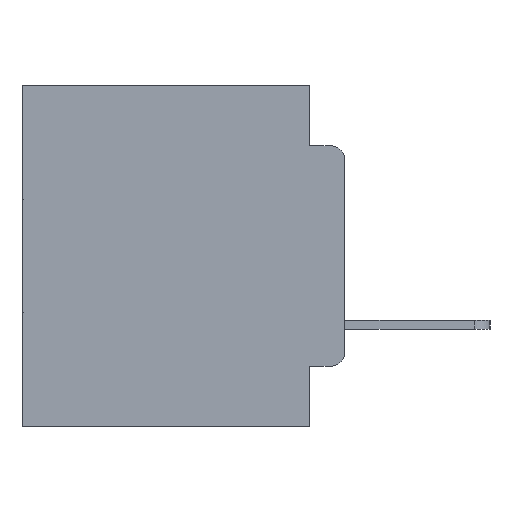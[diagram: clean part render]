
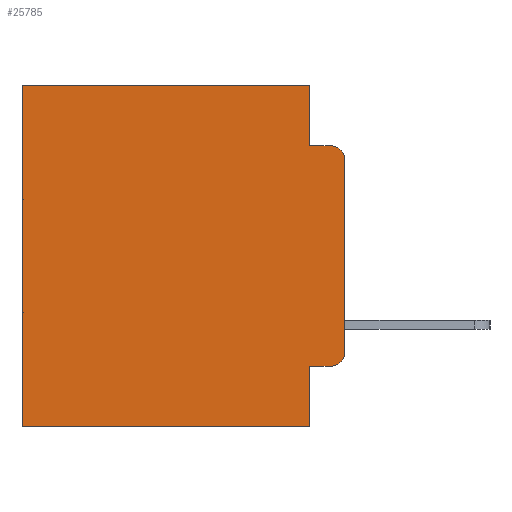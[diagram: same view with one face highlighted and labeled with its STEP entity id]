
A CAD part, left-side view. The second image highlights one B-rep face of the part: STEP entity #25785.
In plain terms, the highlighted planar face has unit normal (-1, 0, 0).
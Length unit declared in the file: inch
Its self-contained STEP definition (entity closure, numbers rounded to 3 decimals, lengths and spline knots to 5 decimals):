
#157 = CARTESIAN_POINT ( 'NONE',  ( 0.298, 0., -0.3915 ) ) ;
#296 = AXIS2_PLACEMENT_3D ( 'NONE', #23354, #9977, #25510 ) ;
#390 = DIRECTION ( 'NONE',  ( 1., 0., 0. ) ) ;
#1277 = LINE ( 'NONE', #17459, #25351 ) ;
#1589 = DIRECTION ( 'NONE',  ( 0., -1., 0. ) ) ;
#1739 = LINE ( 'NONE', #18466, #7042 ) ;
#2815 = ORIENTED_EDGE ( 'NONE', *, *, #13918, .F. ) ;
#3481 = FACE_OUTER_BOUND ( 'NONE', #18692, .T. ) ;
#3540 = CARTESIAN_POINT ( 'NONE',  ( 0.298, 0.051, 0. ) ) ;
#3542 = EDGE_CURVE ( 'NONE', #17541, #8815, #22103, .T. ) ;
#3985 = ORIENTED_EDGE ( 'NONE', *, *, #18609, .T. ) ;
#4262 = ORIENTED_EDGE ( 'NONE', *, *, #20008, .F. ) ;
#4899 = ORIENTED_EDGE ( 'NONE', *, *, #21654, .F. ) ;
#5391 = CARTESIAN_POINT ( 'NONE',  ( 0.298, 0.02, -0.1085 ) ) ;
#5710 = ORIENTED_EDGE ( 'NONE', *, *, #10052, .T. ) ;
#6022 = LINE ( 'NONE', #25592, #12409 ) ;
#6202 = ORIENTED_EDGE ( 'NONE', *, *, #3542, .T. ) ;
#6650 = ORIENTED_EDGE ( 'NONE', *, *, #12881, .F. ) ;
#7029 = ORIENTED_EDGE ( 'NONE', *, *, #26324, .F. ) ;
#7042 = VECTOR ( 'NONE', #18252, 39.37008 ) ;
#7412 = ORIENTED_EDGE ( 'NONE', *, *, #27875, .T. ) ;
#7797 = ORIENTED_EDGE ( 'NONE', *, *, #28250, .T. ) ;
#7899 = DIRECTION ( 'NONE',  ( 0., 0., -1. ) ) ;
#8348 = CARTESIAN_POINT ( 'NONE',  ( 0.298, 0., -0.5 ) ) ;
#8815 = VERTEX_POINT ( 'NONE', #25497 ) ;
#8948 = VERTEX_POINT ( 'NONE', #21091 ) ;
#9608 = AXIS2_PLACEMENT_3D ( 'NONE', #5391, #21474, #7899 ) ;
#9977 = DIRECTION ( 'NONE',  ( -1., 0., 0. ) ) ;
#10052 = EDGE_CURVE ( 'NONE', #25982, #17541, #1739, .T. ) ;
#10218 = VECTOR ( 'NONE', #15419, 39.37008 ) ;
#10596 = CARTESIAN_POINT ( 'NONE',  ( 0.298, 0., 0. ) ) ;
#10712 = CARTESIAN_POINT ( 'NONE',  ( 0.298, 0.02, -0.4115 ) ) ;
#10760 = DIRECTION ( 'NONE',  ( 0., 1., 0. ) ) ;
#11205 = VECTOR ( 'NONE', #17823, 39.37008 ) ;
#11633 = CARTESIAN_POINT ( 'NONE',  ( 0.298, 0.02, -0.0885 ) ) ;
#11638 = VERTEX_POINT ( 'NONE', #27804 ) ;
#12241 = CARTESIAN_POINT ( 'NONE',  ( 0.298, 0.051, -0.5 ) ) ;
#12368 = VERTEX_POINT ( 'NONE', #157 ) ;
#12409 = VECTOR ( 'NONE', #14722, 39.37008 ) ;
#12881 = EDGE_CURVE ( 'NONE', #21218, #8815, #27850, .T. ) ;
#13629 = VERTEX_POINT ( 'NONE', #11633 ) ;
#13918 = EDGE_CURVE ( 'NONE', #11638, #12368, #15969, .T. ) ;
#14309 = LINE ( 'NONE', #28973, #25235 ) ;
#14722 = DIRECTION ( 'NONE',  ( 0., 0., -1. ) ) ;
#15110 = DIRECTION ( 'NONE',  ( 0., 0., -1. ) ) ;
#15409 = CARTESIAN_POINT ( 'NONE',  ( 0.298, 0.473, 0. ) ) ;
#15419 = DIRECTION ( 'NONE',  ( 0., 0., -1. ) ) ;
#15969 = LINE ( 'NONE', #10596, #21771 ) ;
#16359 = VERTEX_POINT ( 'NONE', #24412 ) ;
#16387 = VECTOR ( 'NONE', #10760, 39.37008 ) ;
#17242 = LINE ( 'NONE', #3540, #11205 ) ;
#17357 = DIRECTION ( 'NONE',  ( 0., 0., -1. ) ) ;
#17459 = CARTESIAN_POINT ( 'NONE',  ( 0.298, 0.051, -0.4115 ) ) ;
#17541 = VERTEX_POINT ( 'NONE', #27069 ) ;
#17823 = DIRECTION ( 'NONE',  ( 0., 0., -1. ) ) ;
#18252 = DIRECTION ( 'NONE',  ( 0., 1., 0. ) ) ;
#18466 = CARTESIAN_POINT ( 'NONE',  ( 0.298, 0., 0. ) ) ;
#18609 = EDGE_CURVE ( 'NONE', #11638, #13629, #21934, .T. ) ;
#18692 = EDGE_LOOP ( 'NONE', ( #2815, #3985, #4262, #4899, #5710, #6202, #6650, #7029, #7412, #7797 ) ) ;
#20008 = EDGE_CURVE ( 'NONE', #8948, #13629, #14309, .T. ) ;
#21091 = CARTESIAN_POINT ( 'NONE',  ( 0.298, 0.051, -0.0885 ) ) ;
#21218 = VERTEX_POINT ( 'NONE', #12241 ) ;
#21474 = DIRECTION ( 'NONE',  ( -1., 0., 0. ) ) ;
#21654 = EDGE_CURVE ( 'NONE', #25982, #8948, #17242, .T. ) ;
#21771 = VECTOR ( 'NONE', #15110, 39.37008 ) ;
#21934 = CIRCLE ( 'NONE', #9608, 0.02 ) ;
#22103 = LINE ( 'NONE', #15409, #10218 ) ;
#22206 = CARTESIAN_POINT ( 'NONE',  ( 0.298, 0.051, 0. ) ) ;
#23354 = CARTESIAN_POINT ( 'NONE',  ( 0.298, 0.02, -0.3915 ) ) ;
#24006 = DIRECTION ( 'NONE',  ( 0., -1., 0. ) ) ;
#24253 = AXIS2_PLACEMENT_3D ( 'NONE', #26007, #390, #17357 ) ;
#24412 = CARTESIAN_POINT ( 'NONE',  ( 0.298, 0.051, -0.4115 ) ) ;
#25235 = VECTOR ( 'NONE', #1589, 39.37008 ) ;
#25351 = VECTOR ( 'NONE', #24006, 39.37008 ) ;
#25497 = CARTESIAN_POINT ( 'NONE',  ( 0.298, 0.473, -0.5 ) ) ;
#25510 = DIRECTION ( 'NONE',  ( 0., 0., -1. ) ) ;
#25592 = CARTESIAN_POINT ( 'NONE',  ( 0.298, 0.051, 0. ) ) ;
#25785 = ADVANCED_FACE ( 'NONE', ( #3481 ), #25907, .F. ) ;
#25907 = PLANE ( 'NONE',  #24253 ) ;
#25982 = VERTEX_POINT ( 'NONE', #22206 ) ;
#26007 = CARTESIAN_POINT ( 'NONE',  ( 0.298, 0., 0. ) ) ;
#26324 = EDGE_CURVE ( 'NONE', #16359, #21218, #6022, .T. ) ;
#27069 = CARTESIAN_POINT ( 'NONE',  ( 0.298, 0.473, 0. ) ) ;
#27804 = CARTESIAN_POINT ( 'NONE',  ( 0.298, 0., -0.1085 ) ) ;
#27850 = LINE ( 'NONE', #8348, #16387 ) ;
#27875 = EDGE_CURVE ( 'NONE', #16359, #27902, #1277, .T. ) ;
#27902 = VERTEX_POINT ( 'NONE', #10712 ) ;
#27942 = CIRCLE ( 'NONE', #296, 0.02 ) ;
#28250 = EDGE_CURVE ( 'NONE', #27902, #12368, #27942, .T. ) ;
#28973 = CARTESIAN_POINT ( 'NONE',  ( 0.298, 0.051, -0.0885 ) ) ;
